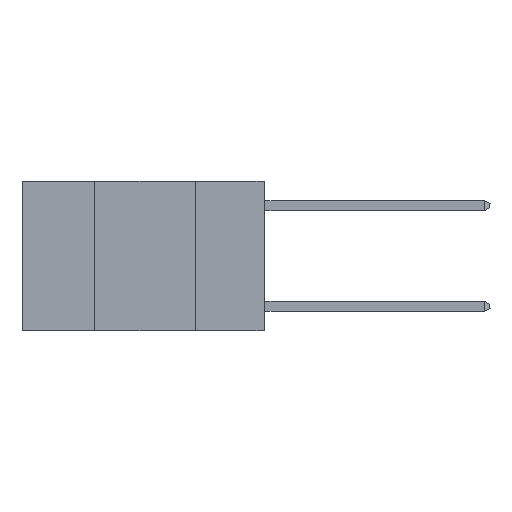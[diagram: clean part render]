
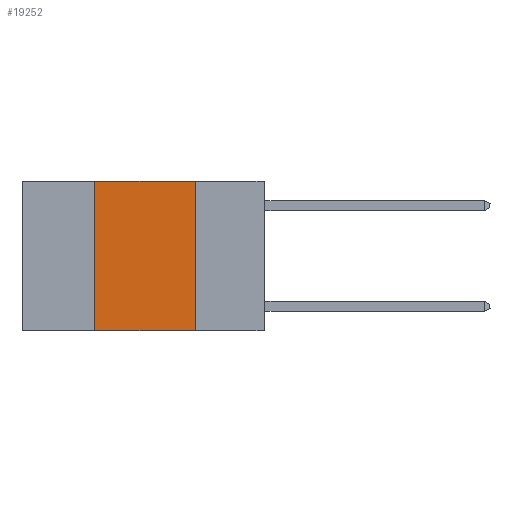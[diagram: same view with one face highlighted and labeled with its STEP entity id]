
A CAD part, left-side view. The second image highlights one B-rep face of the part: STEP entity #19252.
In plain terms, the highlighted planar face has unit normal (-1, 0, 0).
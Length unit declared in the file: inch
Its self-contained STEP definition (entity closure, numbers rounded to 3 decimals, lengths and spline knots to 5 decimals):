
#776 = CARTESIAN_POINT ( 'NONE',  ( 0., 0.17, 0. ) ) ;
#1372 = CARTESIAN_POINT ( 'NONE',  ( 0., 0.6, -0.37 ) ) ;
#2516 = CARTESIAN_POINT ( 'NONE',  ( 0., 0.42, -0.37 ) ) ;
#3030 = EDGE_CURVE ( 'NONE', #7297, #15630, #14472, .T. ) ;
#6099 = FACE_OUTER_BOUND ( 'NONE', #12716, .T. ) ;
#6287 = VERTEX_POINT ( 'NONE', #776 ) ;
#6855 = LINE ( 'NONE', #11569, #17027 ) ;
#7297 = VERTEX_POINT ( 'NONE', #2516 ) ;
#8180 = ORIENTED_EDGE ( 'NONE', *, *, #18539, .F. ) ;
#8252 = DIRECTION ( 'NONE',  ( 0., 0., 1. ) ) ;
#8415 = CARTESIAN_POINT ( 'NONE',  ( 0., 0.17, -0.37 ) ) ;
#9033 = PLANE ( 'NONE',  #16128 ) ;
#9319 = CARTESIAN_POINT ( 'NONE',  ( 0., 0.42, 0. ) ) ;
#9626 = CARTESIAN_POINT ( 'NONE',  ( 0., 0.42, 0. ) ) ;
#10361 = DIRECTION ( 'NONE',  ( 0., 0., -1. ) ) ;
#11486 = VERTEX_POINT ( 'NONE', #8415 ) ;
#11569 = CARTESIAN_POINT ( 'NONE',  ( 0., 0.6, 0. ) ) ;
#12445 = ORIENTED_EDGE ( 'NONE', *, *, #14800, .F. ) ;
#12500 = ORIENTED_EDGE ( 'NONE', *, *, #3030, .F. ) ;
#12716 = EDGE_LOOP ( 'NONE', ( #8180, #12445, #12500, #18799 ) ) ;
#13558 = DIRECTION ( 'NONE',  ( 1., 0., 0. ) ) ;
#13739 = LINE ( 'NONE', #1372, #18278 ) ;
#14025 = EDGE_CURVE ( 'NONE', #7297, #11486, #13739, .T. ) ;
#14472 = LINE ( 'NONE', #9626, #15788 ) ;
#14607 = LINE ( 'NONE', #16188, #17712 ) ;
#14800 = EDGE_CURVE ( 'NONE', #15630, #6287, #6855, .T. ) ;
#15630 = VERTEX_POINT ( 'NONE', #9319 ) ;
#15788 = VECTOR ( 'NONE', #8252, 39.37008 ) ;
#16128 = AXIS2_PLACEMENT_3D ( 'NONE', #18372, #13558, #19673 ) ;
#16188 = CARTESIAN_POINT ( 'NONE',  ( 0., 0.17, 0. ) ) ;
#16635 = DIRECTION ( 'NONE',  ( 0., -1., 0. ) ) ;
#17027 = VECTOR ( 'NONE', #19218, 39.37008 ) ;
#17712 = VECTOR ( 'NONE', #10361, 39.37008 ) ;
#18278 = VECTOR ( 'NONE', #16635, 39.37008 ) ;
#18372 = CARTESIAN_POINT ( 'NONE',  ( 0., 0.6, 0. ) ) ;
#18539 = EDGE_CURVE ( 'NONE', #6287, #11486, #14607, .T. ) ;
#18799 = ORIENTED_EDGE ( 'NONE', *, *, #14025, .T. ) ;
#19218 = DIRECTION ( 'NONE',  ( 0., -1., 0. ) ) ;
#19252 = ADVANCED_FACE ( 'NONE', ( #6099 ), #9033, .F. ) ;
#19673 = DIRECTION ( 'NONE',  ( 0., 0., -1. ) ) ;
